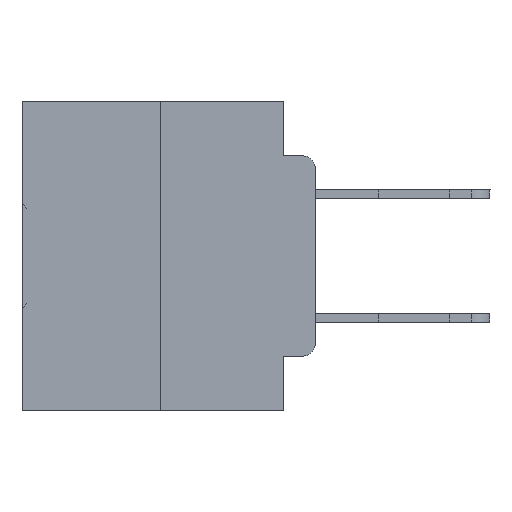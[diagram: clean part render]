
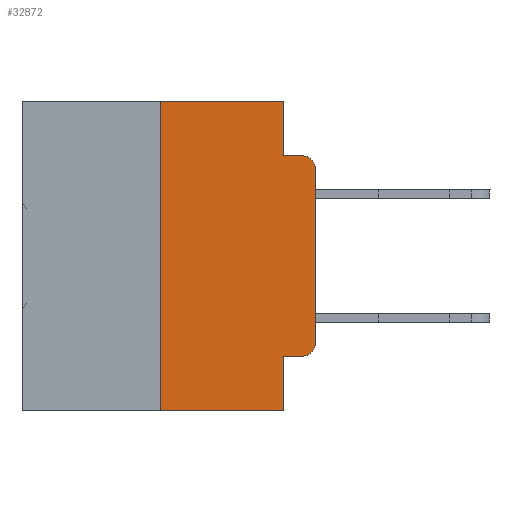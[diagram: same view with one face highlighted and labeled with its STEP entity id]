
A CAD part, left-side view. The second image highlights one B-rep face of the part: STEP entity #32872.
In plain terms, the highlighted planar face has unit normal (-1, 0, 0).
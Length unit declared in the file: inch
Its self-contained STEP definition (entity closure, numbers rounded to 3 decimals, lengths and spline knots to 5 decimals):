
#18 = EDGE_CURVE ( 'NONE', #16889, #27100, #30153, .T. ) ;
#633 = DIRECTION ( 'NONE',  ( 0., -1., 0. ) ) ;
#706 = PLANE ( 'NONE',  #18163 ) ;
#2831 = CARTESIAN_POINT ( 'NONE',  ( 0., 0.051, 0. ) ) ;
#3954 = DIRECTION ( 'NONE',  ( -1., 0., 0. ) ) ;
#4322 = DIRECTION ( 'NONE',  ( -1., 0., 0. ) ) ;
#4344 = AXIS2_PLACEMENT_3D ( 'NONE', #17377, #3954, #33426 ) ;
#5087 = LINE ( 'NONE', #26348, #21242 ) ;
#5531 = CARTESIAN_POINT ( 'NONE',  ( 0., 0., -0.1085 ) ) ;
#5902 = CARTESIAN_POINT ( 'NONE',  ( 0., 0.02, -0.0885 ) ) ;
#5904 = LINE ( 'NONE', #29988, #34525 ) ;
#5979 = DIRECTION ( 'NONE',  ( 1., 0., 0. ) ) ;
#6089 = VECTOR ( 'NONE', #20939, 39.37008 ) ;
#6737 = CARTESIAN_POINT ( 'NONE',  ( 0., 0.051, -0.0885 ) ) ;
#6875 = CARTESIAN_POINT ( 'NONE',  ( 0., 0.473, -0.5 ) ) ;
#7541 = CARTESIAN_POINT ( 'NONE',  ( 0., 0., -0.3915 ) ) ;
#8154 = ORIENTED_EDGE ( 'NONE', *, *, #18, .T. ) ;
#8413 = CARTESIAN_POINT ( 'NONE',  ( 0., 0.051, -0.4115 ) ) ;
#9302 = VERTEX_POINT ( 'NONE', #6737 ) ;
#10467 = VERTEX_POINT ( 'NONE', #29630 ) ;
#10489 = ORIENTED_EDGE ( 'NONE', *, *, #29916, .F. ) ;
#12748 = AXIS2_PLACEMENT_3D ( 'NONE', #18178, #4322, #12924 ) ;
#12924 = DIRECTION ( 'NONE',  ( 0., 0., -1. ) ) ;
#13759 = DIRECTION ( 'NONE',  ( 0., 0., 1. ) ) ;
#13903 = VECTOR ( 'NONE', #13759, 39.37008 ) ;
#14188 = ORIENTED_EDGE ( 'NONE', *, *, #26669, .F. ) ;
#14622 = VERTEX_POINT ( 'NONE', #7541 ) ;
#14774 = VERTEX_POINT ( 'NONE', #27221 ) ;
#15620 = VECTOR ( 'NONE', #16437, 39.37008 ) ;
#15880 = EDGE_CURVE ( 'NONE', #10467, #9302, #5087, .T. ) ;
#16291 = ORIENTED_EDGE ( 'NONE', *, *, #23468, .F. ) ;
#16437 = DIRECTION ( 'NONE',  ( 0., 0., 1. ) ) ;
#16610 = LINE ( 'NONE', #27153, #15620 ) ;
#16889 = VERTEX_POINT ( 'NONE', #5531 ) ;
#16895 = VERTEX_POINT ( 'NONE', #30587 ) ;
#17302 = VERTEX_POINT ( 'NONE', #8413 ) ;
#17377 = CARTESIAN_POINT ( 'NONE',  ( 0., 0.02, -0.1085 ) ) ;
#17885 = EDGE_CURVE ( 'NONE', #14774, #16895, #23225, .T. ) ;
#18083 = DIRECTION ( 'NONE',  ( 0., -1., 0. ) ) ;
#18163 = AXIS2_PLACEMENT_3D ( 'NONE', #19165, #5979, #19002 ) ;
#18178 = CARTESIAN_POINT ( 'NONE',  ( 0., 0.02, -0.3915 ) ) ;
#18249 = LINE ( 'NONE', #28967, #25297 ) ;
#18278 = VERTEX_POINT ( 'NONE', #25136 ) ;
#18636 = FACE_OUTER_BOUND ( 'NONE', #21039, .T. ) ;
#19002 = DIRECTION ( 'NONE',  ( 0., 0., -1. ) ) ;
#19165 = CARTESIAN_POINT ( 'NONE',  ( 0., 0.473, 0. ) ) ;
#20432 = ORIENTED_EDGE ( 'NONE', *, *, #24360, .T. ) ;
#20562 = VERTEX_POINT ( 'NONE', #25904 ) ;
#20939 = DIRECTION ( 'NONE',  ( 0., -1., 0. ) ) ;
#21039 = EDGE_LOOP ( 'NONE', ( #20432, #8154, #10489, #21808, #14188, #16291, #21584, #34569, #27575, #31797 ) ) ;
#21242 = VECTOR ( 'NONE', #29341, 39.37008 ) ;
#21483 = CARTESIAN_POINT ( 'NONE',  ( 0., 0.25, 0. ) ) ;
#21571 = EDGE_CURVE ( 'NONE', #18278, #14622, #31271, .T. ) ;
#21584 = ORIENTED_EDGE ( 'NONE', *, *, #17885, .T. ) ;
#21794 = DIRECTION ( 'NONE',  ( 0., 0., -1. ) ) ;
#21808 = ORIENTED_EDGE ( 'NONE', *, *, #15880, .F. ) ;
#22894 = VECTOR ( 'NONE', #21794, 39.37008 ) ;
#23225 = LINE ( 'NONE', #6875, #6089 ) ;
#23468 = EDGE_CURVE ( 'NONE', #14774, #20562, #31838, .T. ) ;
#23949 = EDGE_CURVE ( 'NONE', #17302, #16895, #29349, .T. ) ;
#24360 = EDGE_CURVE ( 'NONE', #14622, #16889, #16610, .T. ) ;
#25136 = CARTESIAN_POINT ( 'NONE',  ( 0., 0.02, -0.4115 ) ) ;
#25297 = VECTOR ( 'NONE', #18083, 39.37008 ) ;
#25904 = CARTESIAN_POINT ( 'NONE',  ( 0., 0.25, 0. ) ) ;
#26348 = CARTESIAN_POINT ( 'NONE',  ( 0., 0.051, 0. ) ) ;
#26669 = EDGE_CURVE ( 'NONE', #20562, #10467, #18249, .T. ) ;
#27100 = VERTEX_POINT ( 'NONE', #5902 ) ;
#27153 = CARTESIAN_POINT ( 'NONE',  ( 0., 0., 0. ) ) ;
#27221 = CARTESIAN_POINT ( 'NONE',  ( 0., 0.25, -0.5 ) ) ;
#27575 = ORIENTED_EDGE ( 'NONE', *, *, #34504, .T. ) ;
#28967 = CARTESIAN_POINT ( 'NONE',  ( 0., 0.473, 0. ) ) ;
#29306 = DIRECTION ( 'NONE',  ( 0., -1., 0. ) ) ;
#29341 = DIRECTION ( 'NONE',  ( 0., 0., -1. ) ) ;
#29349 = LINE ( 'NONE', #2831, #22894 ) ;
#29630 = CARTESIAN_POINT ( 'NONE',  ( 0., 0.051, 0. ) ) ;
#29916 = EDGE_CURVE ( 'NONE', #9302, #27100, #31938, .T. ) ;
#29988 = CARTESIAN_POINT ( 'NONE',  ( 0., 0.051, -0.4115 ) ) ;
#30153 = CIRCLE ( 'NONE', #4344, 0.02 ) ;
#30587 = CARTESIAN_POINT ( 'NONE',  ( 0., 0.051, -0.5 ) ) ;
#31271 = CIRCLE ( 'NONE', #12748, 0.02 ) ;
#31534 = VECTOR ( 'NONE', #29306, 39.37008 ) ;
#31589 = CARTESIAN_POINT ( 'NONE',  ( 0., 0.051, -0.0885 ) ) ;
#31797 = ORIENTED_EDGE ( 'NONE', *, *, #21571, .T. ) ;
#31838 = LINE ( 'NONE', #21483, #13903 ) ;
#31938 = LINE ( 'NONE', #31589, #31534 ) ;
#32872 = ADVANCED_FACE ( 'NONE', ( #18636 ), #706, .F. ) ;
#33426 = DIRECTION ( 'NONE',  ( 0., 0., -1. ) ) ;
#34504 = EDGE_CURVE ( 'NONE', #17302, #18278, #5904, .T. ) ;
#34525 = VECTOR ( 'NONE', #633, 39.37008 ) ;
#34569 = ORIENTED_EDGE ( 'NONE', *, *, #23949, .F. ) ;
